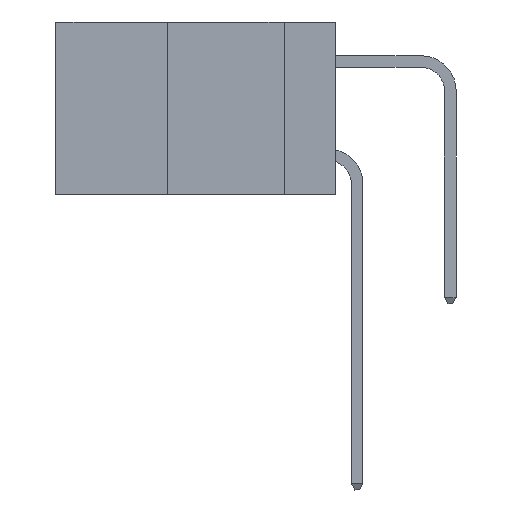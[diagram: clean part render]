
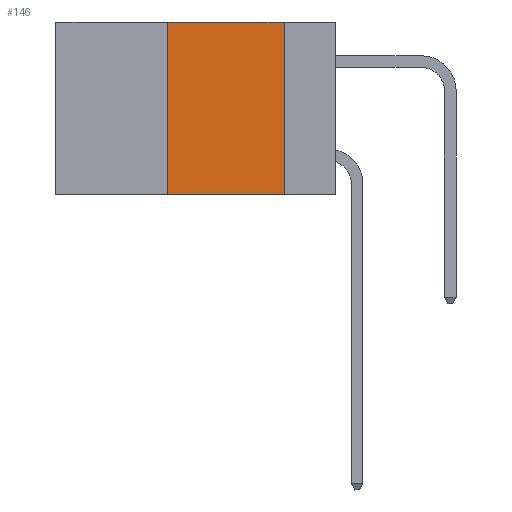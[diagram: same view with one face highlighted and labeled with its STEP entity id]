
A CAD part, left-side view. The second image highlights one B-rep face of the part: STEP entity #146.
In plain terms, the highlighted planar face has unit normal (-1, 0, 0).
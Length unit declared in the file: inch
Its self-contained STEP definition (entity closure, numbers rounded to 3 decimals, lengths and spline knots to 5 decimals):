
#146 = ADVANCED_FACE ( 'NONE', ( #19020 ), #32347, .F. ) ;
#335 = EDGE_LOOP ( 'NONE', ( #7506, #27138, #4207, #27346 ) ) ;
#857 = DIRECTION ( 'NONE',  ( 1., 0., 0. ) ) ;
#2208 = VERTEX_POINT ( 'NONE', #30877 ) ;
#2423 = VERTEX_POINT ( 'NONE', #12739 ) ;
#4207 = ORIENTED_EDGE ( 'NONE', *, *, #10295, .F. ) ;
#4344 = CARTESIAN_POINT ( 'NONE',  ( 0., 0.6, 0. ) ) ;
#6177 = DIRECTION ( 'NONE',  ( 0., 0., 1. ) ) ;
#6843 = VECTOR ( 'NONE', #29912, 39.37008 ) ;
#7176 = CARTESIAN_POINT ( 'NONE',  ( 0., 0.6, -0.37 ) ) ;
#7506 = ORIENTED_EDGE ( 'NONE', *, *, #14220, .F. ) ;
#8396 = LINE ( 'NONE', #14772, #36575 ) ;
#10295 = EDGE_CURVE ( 'NONE', #2208, #14983, #8396, .T. ) ;
#11637 = CARTESIAN_POINT ( 'NONE',  ( 0., 0.11, 0. ) ) ;
#12058 = VECTOR ( 'NONE', #17438, 39.37008 ) ;
#12739 = CARTESIAN_POINT ( 'NONE',  ( 0., 0.11, -0.37 ) ) ;
#13153 = AXIS2_PLACEMENT_3D ( 'NONE', #18453, #857, #21066 ) ;
#14220 = EDGE_CURVE ( 'NONE', #14713, #2423, #34423, .T. ) ;
#14552 = LINE ( 'NONE', #4344, #6843 ) ;
#14713 = VERTEX_POINT ( 'NONE', #19498 ) ;
#14772 = CARTESIAN_POINT ( 'NONE',  ( 0., 0.36, 0. ) ) ;
#14983 = VERTEX_POINT ( 'NONE', #34388 ) ;
#15208 = VECTOR ( 'NONE', #27115, 39.37008 ) ;
#17224 = EDGE_CURVE ( 'NONE', #14983, #14713, #14552, .T. ) ;
#17438 = DIRECTION ( 'NONE',  ( 0., 0., -1. ) ) ;
#18453 = CARTESIAN_POINT ( 'NONE',  ( 0., 0.6, 0. ) ) ;
#19020 = FACE_OUTER_BOUND ( 'NONE', #335, .T. ) ;
#19498 = CARTESIAN_POINT ( 'NONE',  ( 0., 0.11, 0. ) ) ;
#21066 = DIRECTION ( 'NONE',  ( 0., 0., -1. ) ) ;
#27115 = DIRECTION ( 'NONE',  ( 0., -1., 0. ) ) ;
#27138 = ORIENTED_EDGE ( 'NONE', *, *, #17224, .F. ) ;
#27346 = ORIENTED_EDGE ( 'NONE', *, *, #31337, .T. ) ;
#29912 = DIRECTION ( 'NONE',  ( 0., -1., 0. ) ) ;
#30877 = CARTESIAN_POINT ( 'NONE',  ( 0., 0.36, -0.37 ) ) ;
#31337 = EDGE_CURVE ( 'NONE', #2208, #2423, #36569, .T. ) ;
#32347 = PLANE ( 'NONE',  #13153 ) ;
#34388 = CARTESIAN_POINT ( 'NONE',  ( 0., 0.36, 0. ) ) ;
#34423 = LINE ( 'NONE', #11637, #12058 ) ;
#36569 = LINE ( 'NONE', #7176, #15208 ) ;
#36575 = VECTOR ( 'NONE', #6177, 39.37008 ) ;
